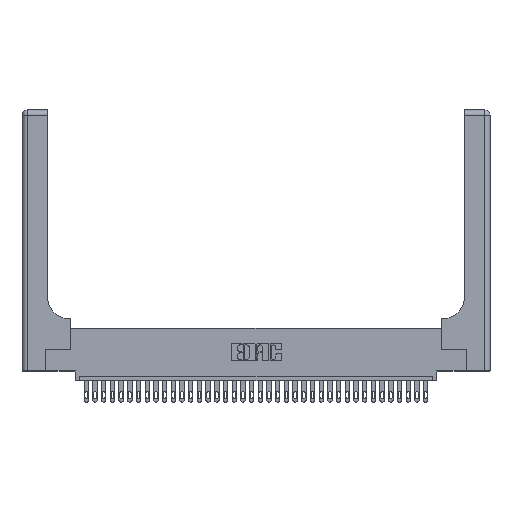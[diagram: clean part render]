
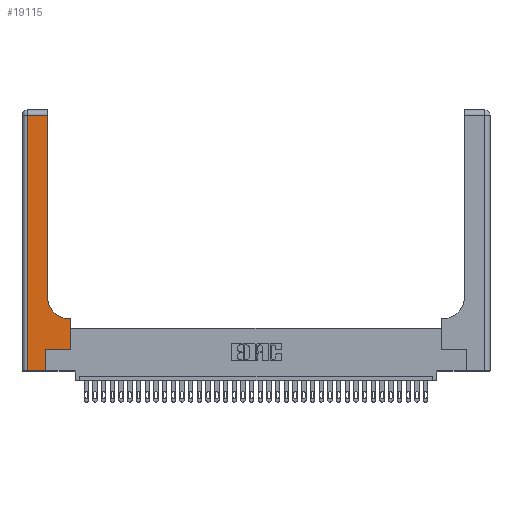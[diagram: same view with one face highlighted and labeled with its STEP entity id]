
A CAD part, top view. The second image highlights one B-rep face of the part: STEP entity #19115.
In plain terms, the highlighted planar face has unit normal (0, 0, 1).
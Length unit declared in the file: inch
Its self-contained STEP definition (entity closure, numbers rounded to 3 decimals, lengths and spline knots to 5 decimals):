
#621 = LINE ( 'NONE', #31110, #29014 ) ;
#852 = ORIENTED_EDGE ( 'NONE', *, *, #29915, .T. ) ;
#1333 = CARTESIAN_POINT ( 'NONE',  ( 0.06, 2.94, 0.37 ) ) ;
#1536 = ORIENTED_EDGE ( 'NONE', *, *, #17969, .T. ) ;
#3545 = VERTEX_POINT ( 'NONE', #1333 ) ;
#4056 = DIRECTION ( 'NONE',  ( -1., 0., 0. ) ) ;
#4904 = VERTEX_POINT ( 'NONE', #20342 ) ;
#5100 = ORIENTED_EDGE ( 'NONE', *, *, #31713, .T. ) ;
#5205 = VERTEX_POINT ( 'NONE', #30252 ) ;
#5586 = DIRECTION ( 'NONE',  ( -1., 0., 0. ) ) ;
#5758 = ORIENTED_EDGE ( 'NONE', *, *, #15637, .T. ) ;
#5826 = DIRECTION ( 'NONE',  ( 1., 0., 0. ) ) ;
#7179 = LINE ( 'NONE', #27448, #8000 ) ;
#7355 = CARTESIAN_POINT ( 'NONE',  ( 0.5415, 0.6, 0.37 ) ) ;
#8000 = VECTOR ( 'NONE', #24833, 39.37008 ) ;
#8205 = VERTEX_POINT ( 'NONE', #32867 ) ;
#8283 = EDGE_LOOP ( 'NONE', ( #16821, #5758, #26930, #852, #1536, #5100, #32956, #22538, #11153 ) ) ;
#9064 = DIRECTION ( 'NONE',  ( 0., 1., 0. ) ) ;
#9358 = CARTESIAN_POINT ( 'NONE',  ( 0., 2.94, 0.37 ) ) ;
#9744 = VERTEX_POINT ( 'NONE', #31349 ) ;
#11153 = ORIENTED_EDGE ( 'NONE', *, *, #32183, .T. ) ;
#11270 = CARTESIAN_POINT ( 'NONE',  ( 0.06, 0., 0.37 ) ) ;
#12515 = PLANE ( 'NONE',  #17987 ) ;
#12589 = EDGE_CURVE ( 'NONE', #3545, #15830, #621, .T. ) ;
#13028 = CARTESIAN_POINT ( 'NONE',  ( 0.269, 0.25, 0.37 ) ) ;
#13933 = DIRECTION ( 'NONE',  ( 1., 0., 0. ) ) ;
#14172 = DIRECTION ( 'NONE',  ( 0., -1., 0. ) ) ;
#14983 = VECTOR ( 'NONE', #25810, 39.37008 ) ;
#15637 = EDGE_CURVE ( 'NONE', #8205, #3545, #34822, .T. ) ;
#15666 = CIRCLE ( 'NONE', #15686, 0.25 ) ;
#15686 = AXIS2_PLACEMENT_3D ( 'NONE', #22128, #19238, #5826 ) ;
#15830 = VERTEX_POINT ( 'NONE', #11270 ) ;
#16299 = VERTEX_POINT ( 'NONE', #32491 ) ;
#16821 = ORIENTED_EDGE ( 'NONE', *, *, #28712, .T. ) ;
#17529 = DIRECTION ( 'NONE',  ( 1., 0., 0. ) ) ;
#17556 = CARTESIAN_POINT ( 'NONE',  ( 0.5585, 0.25, 0.37 ) ) ;
#17969 = EDGE_CURVE ( 'NONE', #4904, #18823, #7179, .T. ) ;
#17987 = AXIS2_PLACEMENT_3D ( 'NONE', #20723, #18054, #4056 ) ;
#18054 = DIRECTION ( 'NONE',  ( 0., 0., -1. ) ) ;
#18823 = VERTEX_POINT ( 'NONE', #13028 ) ;
#19115 = ADVANCED_FACE ( 'NONE', ( #22920 ), #12515, .F. ) ;
#19238 = DIRECTION ( 'NONE',  ( 0., 0., -1. ) ) ;
#19560 = VECTOR ( 'NONE', #9064, 39.37008 ) ;
#19754 = CARTESIAN_POINT ( 'NONE',  ( 0.269, 0.25, 0.37 ) ) ;
#20342 = CARTESIAN_POINT ( 'NONE',  ( 0.269, 0., 0.37 ) ) ;
#20723 = CARTESIAN_POINT ( 'NONE',  ( 0., 3., 0.37 ) ) ;
#21470 = EDGE_CURVE ( 'NONE', #16299, #5205, #34276, .T. ) ;
#22128 = CARTESIAN_POINT ( 'NONE',  ( 0.5415, 0.85, 0.37 ) ) ;
#22538 = ORIENTED_EDGE ( 'NONE', *, *, #26622, .T. ) ;
#22920 = FACE_OUTER_BOUND ( 'NONE', #8283, .T. ) ;
#23092 = VECTOR ( 'NONE', #17529, 39.37008 ) ;
#23561 = LINE ( 'NONE', #30546, #33023 ) ;
#24833 = DIRECTION ( 'NONE',  ( 0., 1., 0. ) ) ;
#25352 = LINE ( 'NONE', #33775, #14983 ) ;
#25810 = DIRECTION ( 'NONE',  ( 0., 1., 0. ) ) ;
#26001 = VECTOR ( 'NONE', #13933, 39.37008 ) ;
#26622 = EDGE_CURVE ( 'NONE', #5205, #31356, #23561, .T. ) ;
#26930 = ORIENTED_EDGE ( 'NONE', *, *, #12589, .T. ) ;
#27417 = VECTOR ( 'NONE', #28588, 39.37008 ) ;
#27448 = CARTESIAN_POINT ( 'NONE',  ( 0.269, 0., 0.37 ) ) ;
#28506 = CARTESIAN_POINT ( 'NONE',  ( 0., 0., 0.37 ) ) ;
#28588 = DIRECTION ( 'NONE',  ( -1., 0., 0. ) ) ;
#28682 = LINE ( 'NONE', #28506, #23092 ) ;
#28712 = EDGE_CURVE ( 'NONE', #9744, #8205, #25352, .T. ) ;
#29014 = VECTOR ( 'NONE', #14172, 39.37008 ) ;
#29915 = EDGE_CURVE ( 'NONE', #15830, #4904, #28682, .T. ) ;
#30252 = CARTESIAN_POINT ( 'NONE',  ( 0.5585, 0.6, 0.37 ) ) ;
#30546 = CARTESIAN_POINT ( 'NONE',  ( 0.2915, 0.6, 0.37 ) ) ;
#31110 = CARTESIAN_POINT ( 'NONE',  ( 0.06, 3., 0.37 ) ) ;
#31349 = CARTESIAN_POINT ( 'NONE',  ( 0.2915, 0.85, 0.37 ) ) ;
#31356 = VERTEX_POINT ( 'NONE', #7355 ) ;
#31713 = EDGE_CURVE ( 'NONE', #18823, #16299, #32885, .T. ) ;
#32183 = EDGE_CURVE ( 'NONE', #31356, #9744, #15666, .T. ) ;
#32491 = CARTESIAN_POINT ( 'NONE',  ( 0.5585, 0.25, 0.37 ) ) ;
#32867 = CARTESIAN_POINT ( 'NONE',  ( 0.2915, 2.94, 0.37 ) ) ;
#32885 = LINE ( 'NONE', #19754, #26001 ) ;
#32956 = ORIENTED_EDGE ( 'NONE', *, *, #21470, .T. ) ;
#33023 = VECTOR ( 'NONE', #5586, 39.37008 ) ;
#33775 = CARTESIAN_POINT ( 'NONE',  ( 0.2915, 3., 0.37 ) ) ;
#34276 = LINE ( 'NONE', #17556, #19560 ) ;
#34822 = LINE ( 'NONE', #9358, #27417 ) ;
